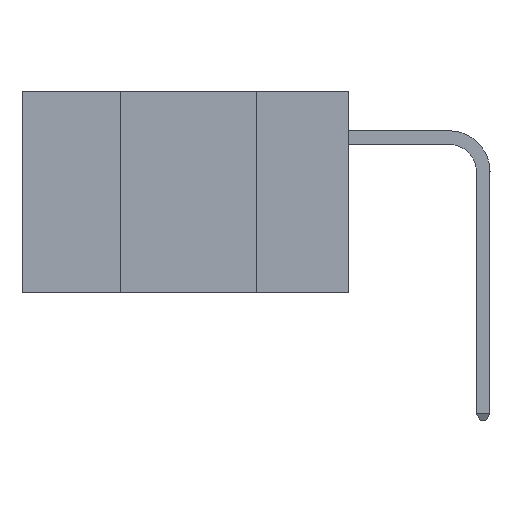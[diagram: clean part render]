
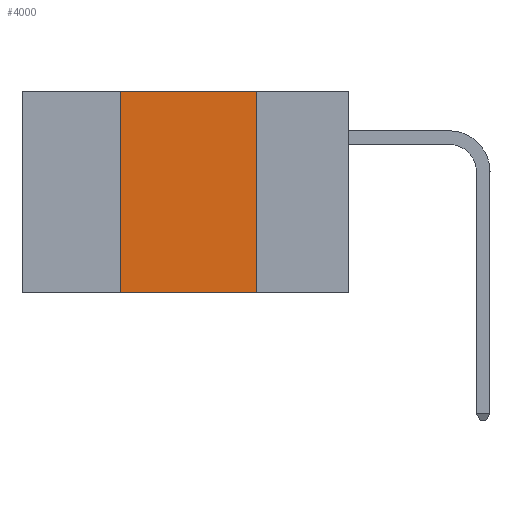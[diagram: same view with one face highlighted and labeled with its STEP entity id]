
A CAD part, left-side view. The second image highlights one B-rep face of the part: STEP entity #4000.
In plain terms, the highlighted planar face has unit normal (-1, 0, 0).
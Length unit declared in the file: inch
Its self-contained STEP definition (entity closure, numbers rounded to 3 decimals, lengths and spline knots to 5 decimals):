
#856 = VERTEX_POINT ( 'NONE', #22070 ) ;
#1232 = LINE ( 'NONE', #1602, #4422 ) ;
#1293 = VECTOR ( 'NONE', #18979, 39.37008 ) ;
#1602 = CARTESIAN_POINT ( 'NONE',  ( 0., 0.42, 0. ) ) ;
#1880 = PLANE ( 'NONE',  #17578 ) ;
#2631 = VERTEX_POINT ( 'NONE', #3235 ) ;
#2748 = LINE ( 'NONE', #14954, #1293 ) ;
#3235 = CARTESIAN_POINT ( 'NONE',  ( 0., 0.42, -0.37 ) ) ;
#4000 = ADVANCED_FACE ( 'NONE', ( #18665 ), #1880, .F. ) ;
#4422 = VECTOR ( 'NONE', #8699, 39.37008 ) ;
#4869 = CARTESIAN_POINT ( 'NONE',  ( 0., 0.17, 0. ) ) ;
#5113 = DIRECTION ( 'NONE',  ( 0., -1., 0. ) ) ;
#6703 = LINE ( 'NONE', #4869, #11393 ) ;
#7481 = ORIENTED_EDGE ( 'NONE', *, *, #18562, .F. ) ;
#8699 = DIRECTION ( 'NONE',  ( 0., 0., 1. ) ) ;
#10287 = CARTESIAN_POINT ( 'NONE',  ( 0., 0.17, -0.37 ) ) ;
#10988 = LINE ( 'NONE', #22140, #23146 ) ;
#11036 = ORIENTED_EDGE ( 'NONE', *, *, #22264, .F. ) ;
#11363 = EDGE_LOOP ( 'NONE', ( #7481, #21012, #11036, #13095 ) ) ;
#11393 = VECTOR ( 'NONE', #18112, 39.37008 ) ;
#11482 = VERTEX_POINT ( 'NONE', #17843 ) ;
#13095 = ORIENTED_EDGE ( 'NONE', *, *, #22725, .T. ) ;
#14954 = CARTESIAN_POINT ( 'NONE',  ( 0., 0.6, 0. ) ) ;
#15429 = CARTESIAN_POINT ( 'NONE',  ( 0., 0.6, 0. ) ) ;
#17153 = DIRECTION ( 'NONE',  ( 0., 0., -1. ) ) ;
#17578 = AXIS2_PLACEMENT_3D ( 'NONE', #15429, #22901, #17153 ) ;
#17843 = CARTESIAN_POINT ( 'NONE',  ( 0., 0.17, 0. ) ) ;
#18112 = DIRECTION ( 'NONE',  ( 0., 0., -1. ) ) ;
#18562 = EDGE_CURVE ( 'NONE', #11482, #20900, #6703, .T. ) ;
#18665 = FACE_OUTER_BOUND ( 'NONE', #11363, .T. ) ;
#18979 = DIRECTION ( 'NONE',  ( 0., -1., 0. ) ) ;
#20900 = VERTEX_POINT ( 'NONE', #10287 ) ;
#21012 = ORIENTED_EDGE ( 'NONE', *, *, #22418, .F. ) ;
#22070 = CARTESIAN_POINT ( 'NONE',  ( 0., 0.42, 0. ) ) ;
#22140 = CARTESIAN_POINT ( 'NONE',  ( 0., 0.6, -0.37 ) ) ;
#22264 = EDGE_CURVE ( 'NONE', #2631, #856, #1232, .T. ) ;
#22418 = EDGE_CURVE ( 'NONE', #856, #11482, #2748, .T. ) ;
#22725 = EDGE_CURVE ( 'NONE', #2631, #20900, #10988, .T. ) ;
#22901 = DIRECTION ( 'NONE',  ( 1., 0., 0. ) ) ;
#23146 = VECTOR ( 'NONE', #5113, 39.37008 ) ;
